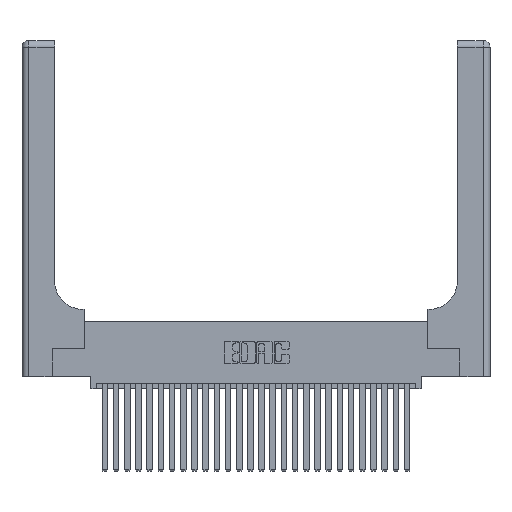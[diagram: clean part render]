
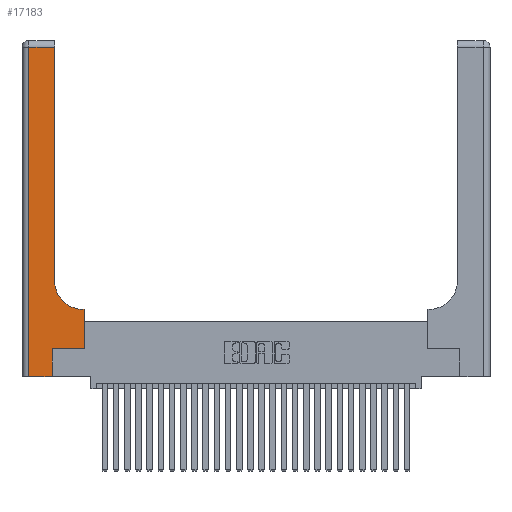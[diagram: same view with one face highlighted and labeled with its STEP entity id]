
A CAD part, top view. The second image highlights one B-rep face of the part: STEP entity #17183.
In plain terms, the highlighted planar face has unit normal (0, 0, 1).
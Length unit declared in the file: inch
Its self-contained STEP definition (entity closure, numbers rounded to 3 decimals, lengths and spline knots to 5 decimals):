
#661 = EDGE_CURVE ( 'NONE', #20573, #13590, #19383, .T. ) ;
#869 = VERTEX_POINT ( 'NONE', #23953 ) ;
#3505 = CARTESIAN_POINT ( 'NONE',  ( 0., 2.94, 0.37 ) ) ;
#3549 = DIRECTION ( 'NONE',  ( 0., 1., 0. ) ) ;
#4023 = VECTOR ( 'NONE', #26824, 39.37008 ) ;
#4202 = CARTESIAN_POINT ( 'NONE',  ( 0.2915, 0.6, 0.37 ) ) ;
#4599 = DIRECTION ( 'NONE',  ( 1., 0., 0. ) ) ;
#4608 = EDGE_CURVE ( 'NONE', #28235, #28013, #20192, .T. ) ;
#4737 = PLANE ( 'NONE',  #10052 ) ;
#5053 = CARTESIAN_POINT ( 'NONE',  ( 0.2915, 0.85, 0.37 ) ) ;
#5731 = DIRECTION ( 'NONE',  ( 0., 0., -1. ) ) ;
#5843 = CARTESIAN_POINT ( 'NONE',  ( 0.06, 0., 0.37 ) ) ;
#6705 = CARTESIAN_POINT ( 'NONE',  ( 0.06, 2.94, 0.37 ) ) ;
#6882 = LINE ( 'NONE', #4202, #24686 ) ;
#7002 = DIRECTION ( 'NONE',  ( 0., 0., -1. ) ) ;
#7753 = CARTESIAN_POINT ( 'NONE',  ( 0.269, 0., 0.37 ) ) ;
#7932 = ORIENTED_EDGE ( 'NONE', *, *, #4608, .T. ) ;
#9043 = CARTESIAN_POINT ( 'NONE',  ( 0.269, 0.25, 0.37 ) ) ;
#9360 = ORIENTED_EDGE ( 'NONE', *, *, #25836, .T. ) ;
#10045 = DIRECTION ( 'NONE',  ( 0., 1., 0. ) ) ;
#10052 = AXIS2_PLACEMENT_3D ( 'NONE', #20457, #7002, #22641 ) ;
#10087 = ORIENTED_EDGE ( 'NONE', *, *, #16864, .T. ) ;
#10474 = LINE ( 'NONE', #7753, #15756 ) ;
#10696 = EDGE_CURVE ( 'NONE', #13590, #28235, #17193, .T. ) ;
#10749 = VECTOR ( 'NONE', #4599, 39.37008 ) ;
#10979 = LINE ( 'NONE', #19317, #11703 ) ;
#11703 = VECTOR ( 'NONE', #3549, 39.37008 ) ;
#12289 = CARTESIAN_POINT ( 'NONE',  ( 0.2915, 3., 0.37 ) ) ;
#12780 = VECTOR ( 'NONE', #25523, 39.37008 ) ;
#12803 = EDGE_CURVE ( 'NONE', #15448, #20573, #13694, .T. ) ;
#13590 = VERTEX_POINT ( 'NONE', #23862 ) ;
#13599 = DIRECTION ( 'NONE',  ( 0., -1., 0. ) ) ;
#13694 = CIRCLE ( 'NONE', #24702, 0.25 ) ;
#13738 = EDGE_CURVE ( 'NONE', #869, #15448, #6882, .T. ) ;
#13853 = EDGE_CURVE ( 'NONE', #26028, #19667, #21257, .T. ) ;
#13983 = ORIENTED_EDGE ( 'NONE', *, *, #26975, .T. ) ;
#15448 = VERTEX_POINT ( 'NONE', #27714 ) ;
#15756 = VECTOR ( 'NONE', #10045, 39.37008 ) ;
#15892 = FACE_OUTER_BOUND ( 'NONE', #27225, .T. ) ;
#16864 = EDGE_CURVE ( 'NONE', #19667, #869, #10979, .T. ) ;
#17183 = ADVANCED_FACE ( 'NONE', ( #15892 ), #4737, .F. ) ;
#17193 = LINE ( 'NONE', #3505, #17885 ) ;
#17885 = VECTOR ( 'NONE', #19276, 39.37008 ) ;
#18186 = VERTEX_POINT ( 'NONE', #20319 ) ;
#18517 = ORIENTED_EDGE ( 'NONE', *, *, #661, .T. ) ;
#19219 = CARTESIAN_POINT ( 'NONE',  ( 0.5415, 0.85, 0.37 ) ) ;
#19276 = DIRECTION ( 'NONE',  ( -1., 0., 0. ) ) ;
#19317 = CARTESIAN_POINT ( 'NONE',  ( 0.5585, 0.25, 0.37 ) ) ;
#19383 = LINE ( 'NONE', #12289, #12780 ) ;
#19547 = CARTESIAN_POINT ( 'NONE',  ( 0.5585, 0.25, 0.37 ) ) ;
#19667 = VERTEX_POINT ( 'NONE', #19547 ) ;
#20192 = LINE ( 'NONE', #28872, #24337 ) ;
#20319 = CARTESIAN_POINT ( 'NONE',  ( 0.269, 0., 0.37 ) ) ;
#20457 = CARTESIAN_POINT ( 'NONE',  ( 0., 3., 0.37 ) ) ;
#20573 = VERTEX_POINT ( 'NONE', #5053 ) ;
#21257 = LINE ( 'NONE', #9043, #4023 ) ;
#21265 = ORIENTED_EDGE ( 'NONE', *, *, #13853, .T. ) ;
#21430 = DIRECTION ( 'NONE',  ( 1., 0., 0. ) ) ;
#22620 = ORIENTED_EDGE ( 'NONE', *, *, #13738, .T. ) ;
#22641 = DIRECTION ( 'NONE',  ( -1., 0., 0. ) ) ;
#23862 = CARTESIAN_POINT ( 'NONE',  ( 0.2915, 2.94, 0.37 ) ) ;
#23953 = CARTESIAN_POINT ( 'NONE',  ( 0.5585, 0.6, 0.37 ) ) ;
#24337 = VECTOR ( 'NONE', #13599, 39.37008 ) ;
#24686 = VECTOR ( 'NONE', #28614, 39.37008 ) ;
#24702 = AXIS2_PLACEMENT_3D ( 'NONE', #19219, #5731, #21430 ) ;
#24735 = CARTESIAN_POINT ( 'NONE',  ( 0., 0., 0.37 ) ) ;
#25037 = ORIENTED_EDGE ( 'NONE', *, *, #10696, .T. ) ;
#25523 = DIRECTION ( 'NONE',  ( 0., 1., 0. ) ) ;
#25836 = EDGE_CURVE ( 'NONE', #18186, #26028, #10474, .T. ) ;
#26028 = VERTEX_POINT ( 'NONE', #28416 ) ;
#26824 = DIRECTION ( 'NONE',  ( 1., 0., 0. ) ) ;
#26975 = EDGE_CURVE ( 'NONE', #28013, #18186, #27012, .T. ) ;
#27012 = LINE ( 'NONE', #24735, #10749 ) ;
#27225 = EDGE_LOOP ( 'NONE', ( #18517, #25037, #7932, #13983, #9360, #21265, #10087, #22620, #28430 ) ) ;
#27714 = CARTESIAN_POINT ( 'NONE',  ( 0.5415, 0.6, 0.37 ) ) ;
#28013 = VERTEX_POINT ( 'NONE', #5843 ) ;
#28235 = VERTEX_POINT ( 'NONE', #6705 ) ;
#28416 = CARTESIAN_POINT ( 'NONE',  ( 0.269, 0.25, 0.37 ) ) ;
#28430 = ORIENTED_EDGE ( 'NONE', *, *, #12803, .T. ) ;
#28614 = DIRECTION ( 'NONE',  ( -1., 0., 0. ) ) ;
#28872 = CARTESIAN_POINT ( 'NONE',  ( 0.06, 3., 0.37 ) ) ;
